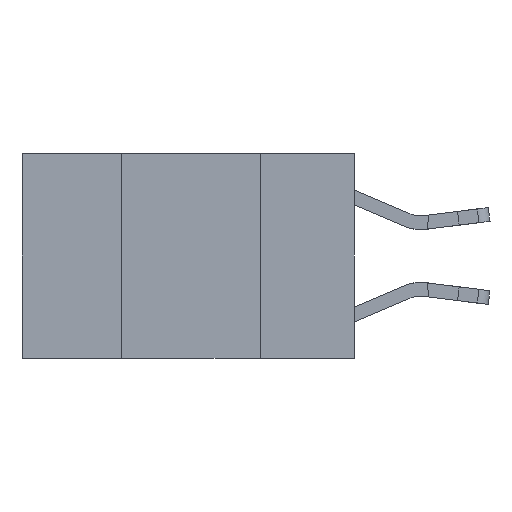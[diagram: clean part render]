
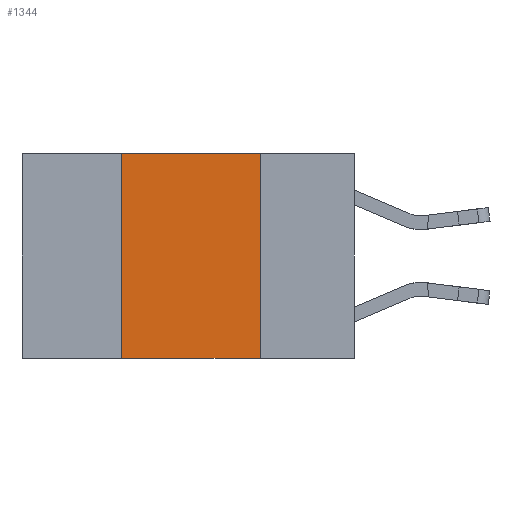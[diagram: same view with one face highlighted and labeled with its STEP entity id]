
A CAD part, left-side view. The second image highlights one B-rep face of the part: STEP entity #1344.
In plain terms, the highlighted planar face has unit normal (-1, 0, 0).
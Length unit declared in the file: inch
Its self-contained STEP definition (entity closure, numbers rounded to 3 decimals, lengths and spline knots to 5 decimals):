
#196 = EDGE_CURVE ( 'NONE', #6788, #8370, #13011, .T. ) ;
#198 = EDGE_CURVE ( 'NONE', #4278, #7236, #6734, .T. ) ;
#223 = EDGE_CURVE ( 'NONE', #4278, #8370, #6381, .T. ) ;
#799 = ORIENTED_EDGE ( 'NONE', *, *, #198, .F. ) ;
#815 = CARTESIAN_POINT ( 'NONE',  ( 0., 0.17, 0. ) ) ;
#907 = DIRECTION ( 'NONE',  ( 0., 0., -1. ) ) ;
#1344 = ADVANCED_FACE ( 'NONE', ( #2926 ), #14381, .F. ) ;
#1726 = EDGE_LOOP ( 'NONE', ( #11742, #8126, #799, #3241 ) ) ;
#2452 = VECTOR ( 'NONE', #14872, 39.37008 ) ;
#2926 = FACE_OUTER_BOUND ( 'NONE', #1726, .T. ) ;
#3241 = ORIENTED_EDGE ( 'NONE', *, *, #223, .T. ) ;
#3385 = VECTOR ( 'NONE', #907, 39.37008 ) ;
#4278 = VERTEX_POINT ( 'NONE', #14609 ) ;
#5418 = CARTESIAN_POINT ( 'NONE',  ( 0., 0.17, 0. ) ) ;
#5437 = CARTESIAN_POINT ( 'NONE',  ( 0., 0.17, -0.37 ) ) ;
#6291 = LINE ( 'NONE', #7828, #2452 ) ;
#6381 = LINE ( 'NONE', #12756, #15039 ) ;
#6618 = DIRECTION ( 'NONE',  ( 0., -1., 0. ) ) ;
#6734 = LINE ( 'NONE', #8540, #12666 ) ;
#6788 = VERTEX_POINT ( 'NONE', #5418 ) ;
#7236 = VERTEX_POINT ( 'NONE', #8542 ) ;
#7717 = AXIS2_PLACEMENT_3D ( 'NONE', #8464, #15554, #8516 ) ;
#7828 = CARTESIAN_POINT ( 'NONE',  ( 0., 0.6, 0. ) ) ;
#8126 = ORIENTED_EDGE ( 'NONE', *, *, #9750, .F. ) ;
#8370 = VERTEX_POINT ( 'NONE', #5437 ) ;
#8464 = CARTESIAN_POINT ( 'NONE',  ( 0., 0.6, 0. ) ) ;
#8516 = DIRECTION ( 'NONE',  ( 0., 0., -1. ) ) ;
#8540 = CARTESIAN_POINT ( 'NONE',  ( 0., 0.42, 0. ) ) ;
#8542 = CARTESIAN_POINT ( 'NONE',  ( 0., 0.42, 0. ) ) ;
#9750 = EDGE_CURVE ( 'NONE', #7236, #6788, #6291, .T. ) ;
#11742 = ORIENTED_EDGE ( 'NONE', *, *, #196, .F. ) ;
#12666 = VECTOR ( 'NONE', #12716, 39.37008 ) ;
#12716 = DIRECTION ( 'NONE',  ( 0., 0., 1. ) ) ;
#12756 = CARTESIAN_POINT ( 'NONE',  ( 0., 0.6, -0.37 ) ) ;
#13011 = LINE ( 'NONE', #815, #3385 ) ;
#14381 = PLANE ( 'NONE',  #7717 ) ;
#14609 = CARTESIAN_POINT ( 'NONE',  ( 0., 0.42, -0.37 ) ) ;
#14872 = DIRECTION ( 'NONE',  ( 0., -1., 0. ) ) ;
#15039 = VECTOR ( 'NONE', #6618, 39.37008 ) ;
#15554 = DIRECTION ( 'NONE',  ( 1., 0., 0. ) ) ;
